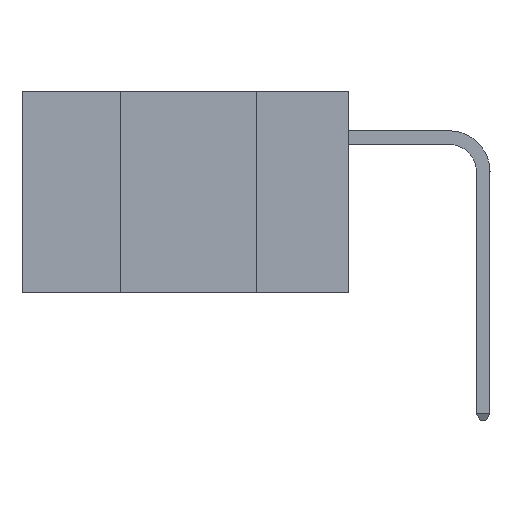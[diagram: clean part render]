
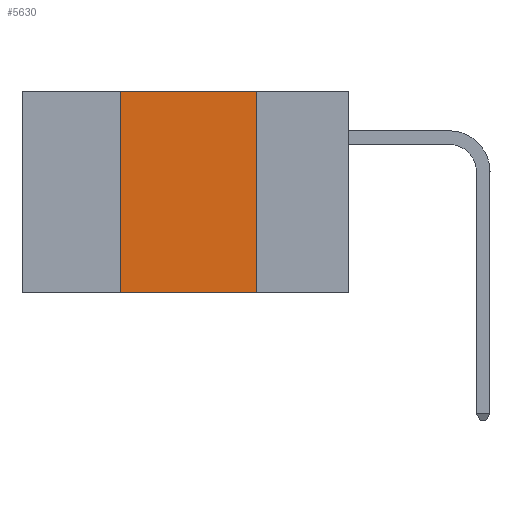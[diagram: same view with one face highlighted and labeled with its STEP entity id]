
A CAD part, left-side view. The second image highlights one B-rep face of the part: STEP entity #5630.
In plain terms, the highlighted planar face has unit normal (-1, 0, 0).
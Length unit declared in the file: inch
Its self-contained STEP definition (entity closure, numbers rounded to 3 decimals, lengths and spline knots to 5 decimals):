
#853 = LINE ( 'NONE', #8136, #3425 ) ;
#1010 = ORIENTED_EDGE ( 'NONE', *, *, #9315, .F. ) ;
#2245 = CARTESIAN_POINT ( 'NONE',  ( 0., 0.17, 0. ) ) ;
#2284 = EDGE_CURVE ( 'NONE', #13555, #6820, #853, .T. ) ;
#2329 = CARTESIAN_POINT ( 'NONE',  ( 0., 0.42, -0.37 ) ) ;
#3056 = LINE ( 'NONE', #10159, #11302 ) ;
#3425 = VECTOR ( 'NONE', #3811, 39.37008 ) ;
#3811 = DIRECTION ( 'NONE',  ( 0., -1., 0. ) ) ;
#3933 = CARTESIAN_POINT ( 'NONE',  ( 0., 0.42, 0. ) ) ;
#4478 = EDGE_CURVE ( 'NONE', #8875, #9139, #12270, .T. ) ;
#5133 = DIRECTION ( 'NONE',  ( 0., 0., -1. ) ) ;
#5299 = VECTOR ( 'NONE', #5133, 39.37008 ) ;
#5630 = ADVANCED_FACE ( 'NONE', ( #11554 ), #11745, .F. ) ;
#6282 = VECTOR ( 'NONE', #8853, 39.37008 ) ;
#6326 = ORIENTED_EDGE ( 'NONE', *, *, #2284, .T. ) ;
#6454 = DIRECTION ( 'NONE',  ( 0., 0., -1. ) ) ;
#6543 = ORIENTED_EDGE ( 'NONE', *, *, #8938, .F. ) ;
#6820 = VERTEX_POINT ( 'NONE', #13476 ) ;
#7812 = CARTESIAN_POINT ( 'NONE',  ( 0., 0.6, 0. ) ) ;
#8136 = CARTESIAN_POINT ( 'NONE',  ( 0., 0.6, -0.37 ) ) ;
#8544 = CARTESIAN_POINT ( 'NONE',  ( 0., 0.6, 0. ) ) ;
#8853 = DIRECTION ( 'NONE',  ( 0., -1., 0. ) ) ;
#8875 = VERTEX_POINT ( 'NONE', #3933 ) ;
#8938 = EDGE_CURVE ( 'NONE', #9139, #6820, #11019, .T. ) ;
#9139 = VERTEX_POINT ( 'NONE', #2245 ) ;
#9315 = EDGE_CURVE ( 'NONE', #13555, #8875, #3056, .T. ) ;
#10089 = ORIENTED_EDGE ( 'NONE', *, *, #4478, .F. ) ;
#10159 = CARTESIAN_POINT ( 'NONE',  ( 0., 0.42, 0. ) ) ;
#11019 = LINE ( 'NONE', #11532, #5299 ) ;
#11217 = DIRECTION ( 'NONE',  ( 0., 0., 1. ) ) ;
#11228 = EDGE_LOOP ( 'NONE', ( #6543, #10089, #1010, #6326 ) ) ;
#11302 = VECTOR ( 'NONE', #11217, 39.37008 ) ;
#11532 = CARTESIAN_POINT ( 'NONE',  ( 0., 0.17, 0. ) ) ;
#11554 = FACE_OUTER_BOUND ( 'NONE', #11228, .T. ) ;
#11745 = PLANE ( 'NONE',  #12225 ) ;
#12225 = AXIS2_PLACEMENT_3D ( 'NONE', #8544, #12788, #6454 ) ;
#12270 = LINE ( 'NONE', #7812, #6282 ) ;
#12788 = DIRECTION ( 'NONE',  ( 1., 0., 0. ) ) ;
#13476 = CARTESIAN_POINT ( 'NONE',  ( 0., 0.17, -0.37 ) ) ;
#13555 = VERTEX_POINT ( 'NONE', #2329 ) ;
